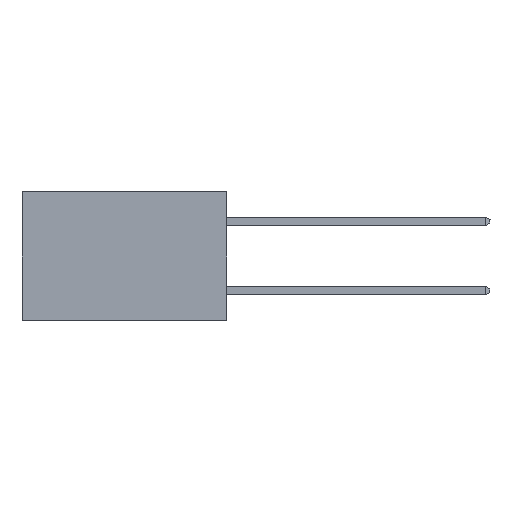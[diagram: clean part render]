
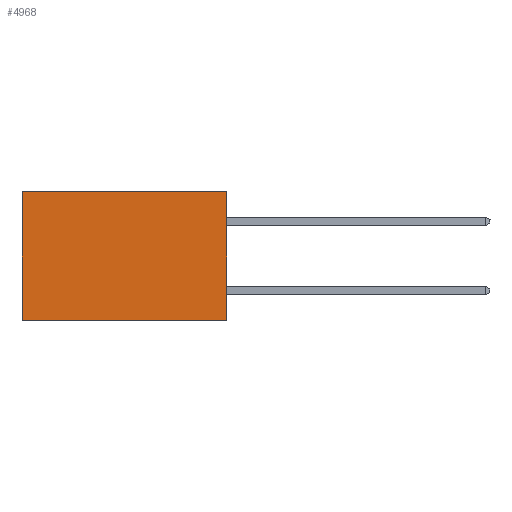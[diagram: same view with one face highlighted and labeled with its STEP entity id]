
A CAD part, left-side view. The second image highlights one B-rep face of the part: STEP entity #4968.
In plain terms, the highlighted planar face has unit normal (-1, 0, 0).
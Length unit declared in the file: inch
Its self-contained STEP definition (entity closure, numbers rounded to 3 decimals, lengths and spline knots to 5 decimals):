
#760 = VERTEX_POINT ( 'NONE', #15271 ) ;
#1670 = VECTOR ( 'NONE', #3035, 39.37008 ) ;
#2485 = EDGE_CURVE ( 'NONE', #15732, #760, #16649, .T. ) ;
#2861 = CARTESIAN_POINT ( 'NONE',  ( 0.277, 0., 0. ) ) ;
#3035 = DIRECTION ( 'NONE',  ( 0., 1., 0. ) ) ;
#4968 = ADVANCED_FACE ( 'NONE', ( #16563 ), #23741, .F. ) ;
#4997 = VERTEX_POINT ( 'NONE', #9244 ) ;
#5646 = EDGE_CURVE ( 'NONE', #15732, #17410, #5901, .T. ) ;
#5901 = LINE ( 'NONE', #20281, #21367 ) ;
#6089 = ORIENTED_EDGE ( 'NONE', *, *, #2485, .T. ) ;
#6349 = VECTOR ( 'NONE', #6475, 39.37008 ) ;
#6475 = DIRECTION ( 'NONE',  ( 0., 1., 0. ) ) ;
#6618 = ORIENTED_EDGE ( 'NONE', *, *, #9203, .F. ) ;
#6841 = CARTESIAN_POINT ( 'NONE',  ( 0.277, 0., -0.37 ) ) ;
#7112 = ORIENTED_EDGE ( 'NONE', *, *, #13050, .T. ) ;
#7492 = LINE ( 'NONE', #16616, #1670 ) ;
#7603 = CARTESIAN_POINT ( 'NONE',  ( 0.277, 0., 0. ) ) ;
#9203 = EDGE_CURVE ( 'NONE', #17410, #4997, #7492, .T. ) ;
#9244 = CARTESIAN_POINT ( 'NONE',  ( 0.277, 0.59, -0.37 ) ) ;
#12823 = DIRECTION ( 'NONE',  ( 0., 0., -1. ) ) ;
#13050 = EDGE_CURVE ( 'NONE', #760, #4997, #20338, .T. ) ;
#13503 = AXIS2_PLACEMENT_3D ( 'NONE', #23109, #22941, #22805 ) ;
#14477 = DIRECTION ( 'NONE',  ( 0., 0., -1. ) ) ;
#15193 = VECTOR ( 'NONE', #14477, 39.37008 ) ;
#15271 = CARTESIAN_POINT ( 'NONE',  ( 0.277, 0.59, 0. ) ) ;
#15732 = VERTEX_POINT ( 'NONE', #7603 ) ;
#16563 = FACE_OUTER_BOUND ( 'NONE', #20696, .T. ) ;
#16616 = CARTESIAN_POINT ( 'NONE',  ( 0.277, 0., -0.37 ) ) ;
#16649 = LINE ( 'NONE', #2861, #6349 ) ;
#17410 = VERTEX_POINT ( 'NONE', #6841 ) ;
#18370 = CARTESIAN_POINT ( 'NONE',  ( 0.277, 0.59, -0.37 ) ) ;
#18759 = ORIENTED_EDGE ( 'NONE', *, *, #5646, .F. ) ;
#20281 = CARTESIAN_POINT ( 'NONE',  ( 0.277, 0., -0.37 ) ) ;
#20338 = LINE ( 'NONE', #18370, #15193 ) ;
#20696 = EDGE_LOOP ( 'NONE', ( #7112, #6618, #18759, #6089 ) ) ;
#21367 = VECTOR ( 'NONE', #12823, 39.37008 ) ;
#22805 = DIRECTION ( 'NONE',  ( 0., 0., -1. ) ) ;
#22941 = DIRECTION ( 'NONE',  ( 1., 0., 0. ) ) ;
#23109 = CARTESIAN_POINT ( 'NONE',  ( 0.277, 0., -0.37 ) ) ;
#23741 = PLANE ( 'NONE',  #13503 ) ;
